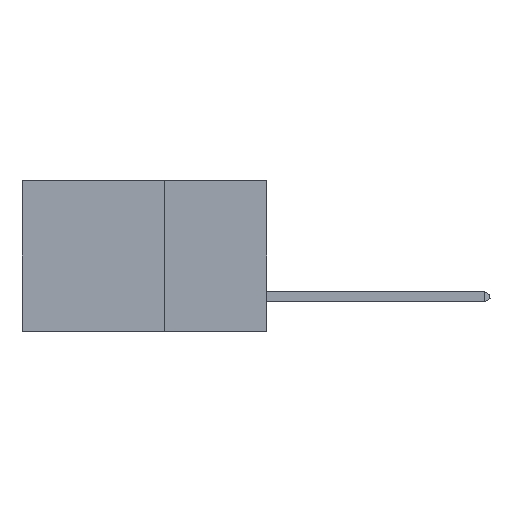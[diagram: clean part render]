
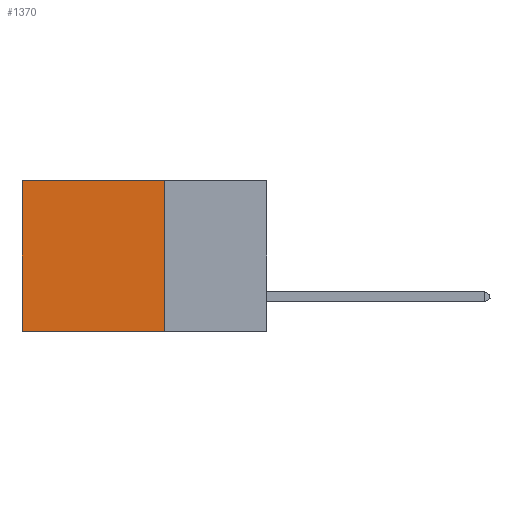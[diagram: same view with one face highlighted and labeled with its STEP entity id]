
A CAD part, left-side view. The second image highlights one B-rep face of the part: STEP entity #1370.
In plain terms, the highlighted planar face has unit normal (-1, 0, 0).
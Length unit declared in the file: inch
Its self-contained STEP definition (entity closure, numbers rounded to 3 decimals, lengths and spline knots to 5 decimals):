
#180 = AXIS2_PLACEMENT_3D ( 'NONE', #3571, #3503, #16230 ) ;
#1370 = ADVANCED_FACE ( 'NONE', ( #1606 ), #13045, .F. ) ;
#1606 = FACE_OUTER_BOUND ( 'NONE', #11752, .T. ) ;
#1719 = ORIENTED_EDGE ( 'NONE', *, *, #15453, .F. ) ;
#2611 = LINE ( 'NONE', #17027, #7330 ) ;
#3238 = DIRECTION ( 'NONE',  ( 0., 1., 0. ) ) ;
#3503 = DIRECTION ( 'NONE',  ( 1., 0., 0. ) ) ;
#3571 = CARTESIAN_POINT ( 'NONE',  ( 0.2875, 0.25, 0. ) ) ;
#4595 = CARTESIAN_POINT ( 'NONE',  ( 0.2875, 0.25, -0.37 ) ) ;
#5070 = VERTEX_POINT ( 'NONE', #20352 ) ;
#6139 = LINE ( 'NONE', #4595, #8886 ) ;
#7330 = VECTOR ( 'NONE', #3238, 39.37008 ) ;
#7334 = LINE ( 'NONE', #20359, #9075 ) ;
#7798 = DIRECTION ( 'NONE',  ( 0., 1., 0. ) ) ;
#7879 = ORIENTED_EDGE ( 'NONE', *, *, #13588, .T. ) ;
#8886 = VECTOR ( 'NONE', #7798, 39.37008 ) ;
#9075 = VECTOR ( 'NONE', #9494, 39.37008 ) ;
#9421 = ORIENTED_EDGE ( 'NONE', *, *, #14133, .F. ) ;
#9494 = DIRECTION ( 'NONE',  ( 0., 0., -1. ) ) ;
#11351 = VERTEX_POINT ( 'NONE', #15704 ) ;
#11721 = EDGE_CURVE ( 'NONE', #12773, #12995, #19819, .T. ) ;
#11752 = EDGE_LOOP ( 'NONE', ( #11898, #1719, #9421, #7879 ) ) ;
#11898 = ORIENTED_EDGE ( 'NONE', *, *, #11721, .T. ) ;
#12773 = VERTEX_POINT ( 'NONE', #15775 ) ;
#12995 = VERTEX_POINT ( 'NONE', #19969 ) ;
#13045 = PLANE ( 'NONE',  #180 ) ;
#13588 = EDGE_CURVE ( 'NONE', #11351, #12773, #2611, .T. ) ;
#13838 = DIRECTION ( 'NONE',  ( 0., 0., -1. ) ) ;
#13921 = VECTOR ( 'NONE', #13838, 39.37008 ) ;
#14133 = EDGE_CURVE ( 'NONE', #11351, #5070, #7334, .T. ) ;
#15453 = EDGE_CURVE ( 'NONE', #5070, #12995, #6139, .T. ) ;
#15492 = CARTESIAN_POINT ( 'NONE',  ( 0.2875, 0.6, 0. ) ) ;
#15704 = CARTESIAN_POINT ( 'NONE',  ( 0.2875, 0.25, 0. ) ) ;
#15775 = CARTESIAN_POINT ( 'NONE',  ( 0.2875, 0.6, 0. ) ) ;
#16230 = DIRECTION ( 'NONE',  ( 0., 0., -1. ) ) ;
#17027 = CARTESIAN_POINT ( 'NONE',  ( 0.2875, 0.25, 0. ) ) ;
#19819 = LINE ( 'NONE', #15492, #13921 ) ;
#19969 = CARTESIAN_POINT ( 'NONE',  ( 0.2875, 0.6, -0.37 ) ) ;
#20352 = CARTESIAN_POINT ( 'NONE',  ( 0.2875, 0.25, -0.37 ) ) ;
#20359 = CARTESIAN_POINT ( 'NONE',  ( 0.2875, 0.25, 0. ) ) ;
